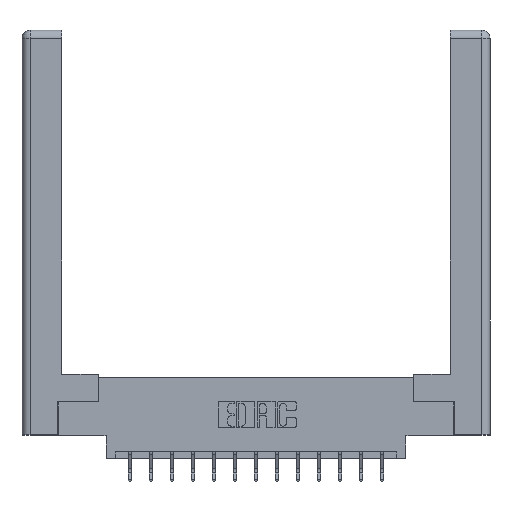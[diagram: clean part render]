
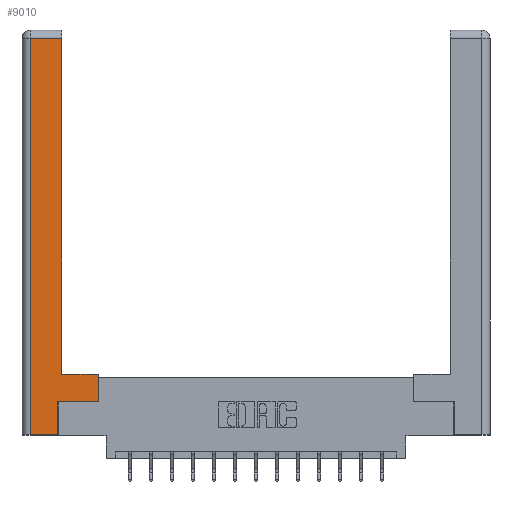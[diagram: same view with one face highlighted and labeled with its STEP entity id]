
A CAD part, top view. The second image highlights one B-rep face of the part: STEP entity #9010.
In plain terms, the highlighted planar face has unit normal (0, 0, 1).
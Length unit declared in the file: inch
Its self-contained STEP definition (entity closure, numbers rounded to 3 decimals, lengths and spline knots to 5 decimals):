
#231 = VERTEX_POINT ( 'NONE', #12213 ) ;
#513 = ORIENTED_EDGE ( 'NONE', *, *, #6386, .T. ) ;
#927 = DIRECTION ( 'NONE',  ( -1., 0., 0. ) ) ;
#1065 = VECTOR ( 'NONE', #5534, 39.37008 ) ;
#1363 = DIRECTION ( 'NONE',  ( 0., 1., 0. ) ) ;
#1459 = LINE ( 'NONE', #15265, #6319 ) ;
#1827 = CARTESIAN_POINT ( 'NONE',  ( 0.295, 2.94, 0. ) ) ;
#1855 = CARTESIAN_POINT ( 'NONE',  ( 0.265, 0.245, 0. ) ) ;
#2345 = VECTOR ( 'NONE', #1363, 39.37008 ) ;
#2506 = EDGE_CURVE ( 'NONE', #4359, #4256, #10226, .T. ) ;
#2685 = LINE ( 'NONE', #11993, #1065 ) ;
#3633 = DIRECTION ( 'NONE',  ( 0., 0., -1. ) ) ;
#4151 = ORIENTED_EDGE ( 'NONE', *, *, #6473, .T. ) ;
#4220 = VERTEX_POINT ( 'NONE', #7901 ) ;
#4221 = LINE ( 'NONE', #14396, #2345 ) ;
#4245 = CARTESIAN_POINT ( 'NONE',  ( 0.565, 0.245, 0. ) ) ;
#4256 = VERTEX_POINT ( 'NONE', #11865 ) ;
#4359 = VERTEX_POINT ( 'NONE', #1827 ) ;
#4843 = DIRECTION ( 'NONE',  ( 1., 0., 0. ) ) ;
#5190 = EDGE_LOOP ( 'NONE', ( #4151, #10302, #11058, #14604, #7090, #513, #8816, #10171 ) ) ;
#5287 = CARTESIAN_POINT ( 'NONE',  ( 0.265, 0.245, 0. ) ) ;
#5534 = DIRECTION ( 'NONE',  ( 0., -1., 0. ) ) ;
#6319 = VECTOR ( 'NONE', #4843, 39.37008 ) ;
#6386 = EDGE_CURVE ( 'NONE', #11300, #16458, #7880, .T. ) ;
#6473 = EDGE_CURVE ( 'NONE', #4220, #4359, #7086, .T. ) ;
#6811 = CARTESIAN_POINT ( 'NONE',  ( 0.565, 0.45, 0. ) ) ;
#7037 = EDGE_CURVE ( 'NONE', #9567, #4220, #12937, .T. ) ;
#7086 = LINE ( 'NONE', #14194, #10495 ) ;
#7090 = ORIENTED_EDGE ( 'NONE', *, *, #7851, .T. ) ;
#7151 = DIRECTION ( 'NONE',  ( 1., 0., 0. ) ) ;
#7656 = EDGE_CURVE ( 'NONE', #16458, #9567, #4221, .T. ) ;
#7851 = EDGE_CURVE ( 'NONE', #10127, #11300, #16451, .T. ) ;
#7880 = LINE ( 'NONE', #4245, #14434 ) ;
#7901 = CARTESIAN_POINT ( 'NONE',  ( 0.295, 0.45, 0. ) ) ;
#8700 = CARTESIAN_POINT ( 'NONE',  ( 0., 0., 0. ) ) ;
#8816 = ORIENTED_EDGE ( 'NONE', *, *, #7656, .T. ) ;
#9010 = ADVANCED_FACE ( 'NONE', ( #10459 ), #10101, .F. ) ;
#9567 = VERTEX_POINT ( 'NONE', #6811 ) ;
#10101 = PLANE ( 'NONE',  #16265 ) ;
#10127 = VERTEX_POINT ( 'NONE', #15809 ) ;
#10171 = ORIENTED_EDGE ( 'NONE', *, *, #7037, .T. ) ;
#10226 = LINE ( 'NONE', #14507, #11463 ) ;
#10302 = ORIENTED_EDGE ( 'NONE', *, *, #2506, .T. ) ;
#10381 = CARTESIAN_POINT ( 'NONE',  ( 0.565, 0.245, 0. ) ) ;
#10459 = FACE_OUTER_BOUND ( 'NONE', #5190, .T. ) ;
#10495 = VECTOR ( 'NONE', #12976, 39.37008 ) ;
#10535 = CARTESIAN_POINT ( 'NONE',  ( 0.295, 0.45, 0. ) ) ;
#10790 = DIRECTION ( 'NONE',  ( 0., 1., 0. ) ) ;
#10910 = EDGE_CURVE ( 'NONE', #4256, #231, #2685, .T. ) ;
#11058 = ORIENTED_EDGE ( 'NONE', *, *, #10910, .T. ) ;
#11300 = VERTEX_POINT ( 'NONE', #5287 ) ;
#11463 = VECTOR ( 'NONE', #15638, 39.37008 ) ;
#11804 = DIRECTION ( 'NONE',  ( -1., 0., 0. ) ) ;
#11865 = CARTESIAN_POINT ( 'NONE',  ( 0.0615, 2.94, 0. ) ) ;
#11993 = CARTESIAN_POINT ( 'NONE',  ( 0.0615, 0., 0. ) ) ;
#12213 = CARTESIAN_POINT ( 'NONE',  ( 0.0615, 0., 0. ) ) ;
#12526 = VECTOR ( 'NONE', #11804, 39.37008 ) ;
#12937 = LINE ( 'NONE', #10535, #12526 ) ;
#12976 = DIRECTION ( 'NONE',  ( 0., 1., 0. ) ) ;
#12996 = EDGE_CURVE ( 'NONE', #231, #10127, #1459, .T. ) ;
#14194 = CARTESIAN_POINT ( 'NONE',  ( 0.295, 3., 0. ) ) ;
#14396 = CARTESIAN_POINT ( 'NONE',  ( 0.565, 0.45, 0. ) ) ;
#14434 = VECTOR ( 'NONE', #7151, 39.37008 ) ;
#14507 = CARTESIAN_POINT ( 'NONE',  ( 0.0615, 2.94, 0. ) ) ;
#14604 = ORIENTED_EDGE ( 'NONE', *, *, #12996, .T. ) ;
#14829 = VECTOR ( 'NONE', #10790, 39.37008 ) ;
#15265 = CARTESIAN_POINT ( 'NONE',  ( 0.265, 0., 0. ) ) ;
#15638 = DIRECTION ( 'NONE',  ( -1., 0., 0. ) ) ;
#15809 = CARTESIAN_POINT ( 'NONE',  ( 0.265, 0., 0. ) ) ;
#16265 = AXIS2_PLACEMENT_3D ( 'NONE', #8700, #3633, #927 ) ;
#16451 = LINE ( 'NONE', #1855, #14829 ) ;
#16458 = VERTEX_POINT ( 'NONE', #10381 ) ;
